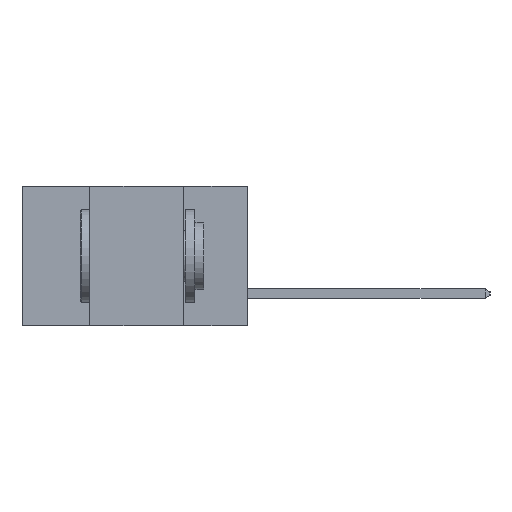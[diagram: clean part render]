
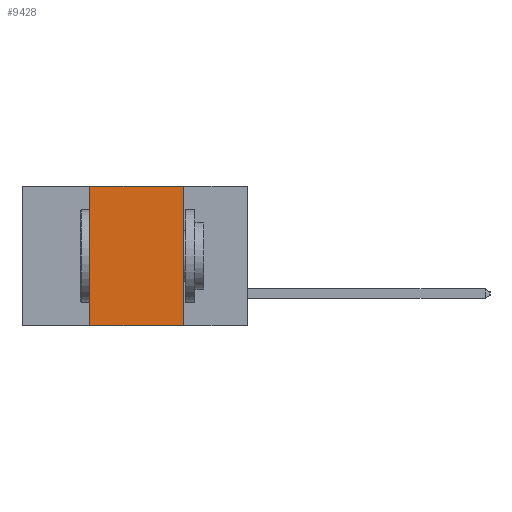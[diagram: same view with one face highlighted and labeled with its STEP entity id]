
A CAD part, left-side view. The second image highlights one B-rep face of the part: STEP entity #9428.
In plain terms, the highlighted planar face has unit normal (-1, 0, 0).
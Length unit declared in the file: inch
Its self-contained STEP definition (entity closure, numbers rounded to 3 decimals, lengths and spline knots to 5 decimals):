
#793 = CARTESIAN_POINT ( 'NONE',  ( 0., 0.17, 0. ) ) ;
#1634 = ORIENTED_EDGE ( 'NONE', *, *, #12651, .F. ) ;
#2711 = VECTOR ( 'NONE', #9846, 39.37008 ) ;
#3221 = VERTEX_POINT ( 'NONE', #4911 ) ;
#3510 = DIRECTION ( 'NONE',  ( 0., 0., -1. ) ) ;
#3540 = DIRECTION ( 'NONE',  ( 1., 0., 0. ) ) ;
#3565 = PLANE ( 'NONE',  #11336 ) ;
#3670 = CARTESIAN_POINT ( 'NONE',  ( 0., 0.6, 0. ) ) ;
#4303 = EDGE_CURVE ( 'NONE', #11898, #22493, #12912, .T. ) ;
#4911 = CARTESIAN_POINT ( 'NONE',  ( 0., 0.17, 0. ) ) ;
#5084 = FACE_OUTER_BOUND ( 'NONE', #16962, .T. ) ;
#6379 = VECTOR ( 'NONE', #19622, 39.37008 ) ;
#6422 = EDGE_CURVE ( 'NONE', #13510, #3221, #11109, .T. ) ;
#6715 = EDGE_CURVE ( 'NONE', #11898, #13510, #14355, .T. ) ;
#8244 = VECTOR ( 'NONE', #11633, 39.37008 ) ;
#8875 = ORIENTED_EDGE ( 'NONE', *, *, #6422, .F. ) ;
#9191 = VECTOR ( 'NONE', #11914, 39.37008 ) ;
#9319 = ORIENTED_EDGE ( 'NONE', *, *, #6715, .F. ) ;
#9428 = ADVANCED_FACE ( 'NONE', ( #5084 ), #3565, .F. ) ;
#9846 = DIRECTION ( 'NONE',  ( 0., 0., -1. ) ) ;
#10231 = CARTESIAN_POINT ( 'NONE',  ( 0., 0.6, -0.37 ) ) ;
#11109 = LINE ( 'NONE', #19805, #6379 ) ;
#11336 = AXIS2_PLACEMENT_3D ( 'NONE', #3670, #3540, #3510 ) ;
#11633 = DIRECTION ( 'NONE',  ( 0., -1., 0. ) ) ;
#11898 = VERTEX_POINT ( 'NONE', #14802 ) ;
#11914 = DIRECTION ( 'NONE',  ( 0., 0., 1. ) ) ;
#12417 = CARTESIAN_POINT ( 'NONE',  ( 0., 0.42, 0. ) ) ;
#12651 = EDGE_CURVE ( 'NONE', #3221, #22493, #21387, .T. ) ;
#12912 = LINE ( 'NONE', #10231, #8244 ) ;
#13510 = VERTEX_POINT ( 'NONE', #14167 ) ;
#14167 = CARTESIAN_POINT ( 'NONE',  ( 0., 0.42, 0. ) ) ;
#14355 = LINE ( 'NONE', #12417, #9191 ) ;
#14802 = CARTESIAN_POINT ( 'NONE',  ( 0., 0.42, -0.37 ) ) ;
#16544 = CARTESIAN_POINT ( 'NONE',  ( 0., 0.17, -0.37 ) ) ;
#16807 = ORIENTED_EDGE ( 'NONE', *, *, #4303, .T. ) ;
#16962 = EDGE_LOOP ( 'NONE', ( #1634, #8875, #9319, #16807 ) ) ;
#19622 = DIRECTION ( 'NONE',  ( 0., -1., 0. ) ) ;
#19805 = CARTESIAN_POINT ( 'NONE',  ( 0., 0.6, 0. ) ) ;
#21387 = LINE ( 'NONE', #793, #2711 ) ;
#22493 = VERTEX_POINT ( 'NONE', #16544 ) ;
